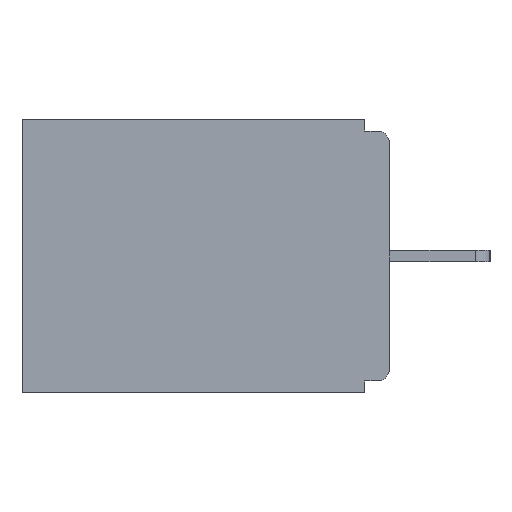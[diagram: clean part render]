
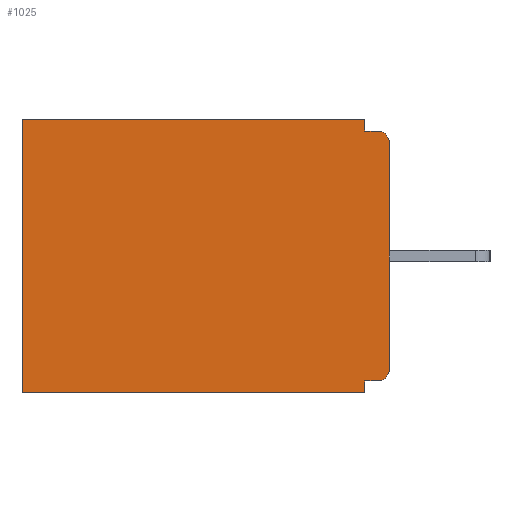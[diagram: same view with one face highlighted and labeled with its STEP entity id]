
A CAD part, left-side view. The second image highlights one B-rep face of the part: STEP entity #1025.
In plain terms, the highlighted planar face has unit normal (-1, 0, 0).
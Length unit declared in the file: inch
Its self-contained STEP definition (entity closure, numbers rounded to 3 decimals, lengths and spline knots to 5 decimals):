
#90 = DIRECTION ( 'NONE',  ( -1., 0., 0. ) ) ;
#140 = VERTEX_POINT ( 'NONE', #8402 ) ;
#780 = PLANE ( 'NONE',  #2413 ) ;
#1025 = ADVANCED_FACE ( 'NONE', ( #2473 ), #780, .F. ) ;
#1148 = ORIENTED_EDGE ( 'NONE', *, *, #9684, .F. ) ;
#1150 = CIRCLE ( 'NONE', #8399, 0.015 ) ;
#1381 = ORIENTED_EDGE ( 'NONE', *, *, #5079, .F. ) ;
#1426 = CARTESIAN_POINT ( 'NONE',  ( 0.298, 0.015, -0.015 ) ) ;
#1466 = CARTESIAN_POINT ( 'NONE',  ( 0.298, 0.46, 0. ) ) ;
#1618 = CARTESIAN_POINT ( 'NONE',  ( 0.298, 0.031, 0. ) ) ;
#1628 = LINE ( 'NONE', #2643, #5589 ) ;
#1726 = DIRECTION ( 'NONE',  ( 0., 0., -1. ) ) ;
#1770 = CARTESIAN_POINT ( 'NONE',  ( 0.298, 0., 0. ) ) ;
#1926 = DIRECTION ( 'NONE',  ( 0., 0., -1. ) ) ;
#1982 = DIRECTION ( 'NONE',  ( 0., 0., -1. ) ) ;
#2405 = EDGE_CURVE ( 'NONE', #10383, #9832, #1628, .T. ) ;
#2413 = AXIS2_PLACEMENT_3D ( 'NONE', #1770, #3349, #8975 ) ;
#2473 = FACE_OUTER_BOUND ( 'NONE', #10370, .T. ) ;
#2510 = VECTOR ( 'NONE', #2753, 39.37008 ) ;
#2528 = LINE ( 'NONE', #3517, #10357 ) ;
#2636 = DIRECTION ( 'NONE',  ( -1., 0., 0. ) ) ;
#2643 = CARTESIAN_POINT ( 'NONE',  ( 0.298, 0., 0. ) ) ;
#2753 = DIRECTION ( 'NONE',  ( 0., 1., 0. ) ) ;
#2997 = VERTEX_POINT ( 'NONE', #1426 ) ;
#3053 = VECTOR ( 'NONE', #3147, 39.37008 ) ;
#3096 = CARTESIAN_POINT ( 'NONE',  ( 0.298, 0.031, -0.343 ) ) ;
#3147 = DIRECTION ( 'NONE',  ( 0., 0., -1. ) ) ;
#3223 = CIRCLE ( 'NONE', #4606, 0.015 ) ;
#3302 = CARTESIAN_POINT ( 'NONE',  ( 0.298, 0.015, -0.313 ) ) ;
#3349 = DIRECTION ( 'NONE',  ( 1., 0., 0. ) ) ;
#3392 = VECTOR ( 'NONE', #7634, 39.37008 ) ;
#3405 = DIRECTION ( 'NONE',  ( 0., 1., 0. ) ) ;
#3458 = DIRECTION ( 'NONE',  ( 0., 0., -1. ) ) ;
#3517 = CARTESIAN_POINT ( 'NONE',  ( 0.298, 0., -0.328 ) ) ;
#3888 = ORIENTED_EDGE ( 'NONE', *, *, #7380, .F. ) ;
#3899 = CARTESIAN_POINT ( 'NONE',  ( 0.298, 0., -0.015 ) ) ;
#3976 = EDGE_CURVE ( 'NONE', #4543, #2997, #9783, .T. ) ;
#4035 = EDGE_CURVE ( 'NONE', #5970, #140, #3223, .T. ) ;
#4049 = CARTESIAN_POINT ( 'NONE',  ( 0.298, 0.015, -0.03 ) ) ;
#4076 = VECTOR ( 'NONE', #8868, 39.37008 ) ;
#4292 = VECTOR ( 'NONE', #1982, 39.37008 ) ;
#4335 = CARTESIAN_POINT ( 'NONE',  ( 0.298, 0.46, 0. ) ) ;
#4396 = EDGE_CURVE ( 'NONE', #5970, #9543, #2528, .T. ) ;
#4543 = VERTEX_POINT ( 'NONE', #5547 ) ;
#4606 = AXIS2_PLACEMENT_3D ( 'NONE', #3302, #2636, #1726 ) ;
#4848 = ORIENTED_EDGE ( 'NONE', *, *, #4035, .T. ) ;
#4960 = VERTEX_POINT ( 'NONE', #5219 ) ;
#5079 = EDGE_CURVE ( 'NONE', #5757, #140, #9377, .T. ) ;
#5086 = DIRECTION ( 'NONE',  ( 0., 1., 0. ) ) ;
#5155 = VECTOR ( 'NONE', #1926, 39.37008 ) ;
#5175 = CARTESIAN_POINT ( 'NONE',  ( 0.298, 0.015, -0.328 ) ) ;
#5198 = ORIENTED_EDGE ( 'NONE', *, *, #9159, .T. ) ;
#5219 = CARTESIAN_POINT ( 'NONE',  ( 0.298, 0.46, -0.343 ) ) ;
#5221 = LINE ( 'NONE', #5334, #5155 ) ;
#5334 = CARTESIAN_POINT ( 'NONE',  ( 0.298, 0.031, -0.343 ) ) ;
#5380 = CARTESIAN_POINT ( 'NONE',  ( 0.298, 0., 0. ) ) ;
#5547 = CARTESIAN_POINT ( 'NONE',  ( 0.298, 0.031, -0.015 ) ) ;
#5589 = VECTOR ( 'NONE', #5086, 39.37008 ) ;
#5757 = VERTEX_POINT ( 'NONE', #6188 ) ;
#5771 = EDGE_CURVE ( 'NONE', #9832, #4960, #7889, .T. ) ;
#5918 = ORIENTED_EDGE ( 'NONE', *, *, #2405, .T. ) ;
#5970 = VERTEX_POINT ( 'NONE', #5175 ) ;
#6044 = CARTESIAN_POINT ( 'NONE',  ( 0.298, 0.031, -0.343 ) ) ;
#6188 = CARTESIAN_POINT ( 'NONE',  ( 0.298, 0., -0.03 ) ) ;
#6507 = CARTESIAN_POINT ( 'NONE',  ( 0.298, 0.031, -0.328 ) ) ;
#6909 = VERTEX_POINT ( 'NONE', #6044 ) ;
#7308 = LINE ( 'NONE', #3096, #3053 ) ;
#7380 = EDGE_CURVE ( 'NONE', #6909, #4960, #7675, .T. ) ;
#7469 = ORIENTED_EDGE ( 'NONE', *, *, #4396, .F. ) ;
#7634 = DIRECTION ( 'NONE',  ( 0., 0., -1. ) ) ;
#7675 = LINE ( 'NONE', #10209, #2510 ) ;
#7889 = LINE ( 'NONE', #4335, #3392 ) ;
#8282 = EDGE_CURVE ( 'NONE', #9543, #6909, #7308, .T. ) ;
#8399 = AXIS2_PLACEMENT_3D ( 'NONE', #4049, #90, #3458 ) ;
#8402 = CARTESIAN_POINT ( 'NONE',  ( 0.298, 0., -0.313 ) ) ;
#8627 = ORIENTED_EDGE ( 'NONE', *, *, #8282, .F. ) ;
#8868 = DIRECTION ( 'NONE',  ( 0., -1., 0. ) ) ;
#8975 = DIRECTION ( 'NONE',  ( 0., 0., -1. ) ) ;
#9159 = EDGE_CURVE ( 'NONE', #5757, #2997, #1150, .T. ) ;
#9377 = LINE ( 'NONE', #5380, #4292 ) ;
#9543 = VERTEX_POINT ( 'NONE', #6507 ) ;
#9587 = ORIENTED_EDGE ( 'NONE', *, *, #5771, .T. ) ;
#9684 = EDGE_CURVE ( 'NONE', #10383, #4543, #5221, .T. ) ;
#9783 = LINE ( 'NONE', #3899, #4076 ) ;
#9832 = VERTEX_POINT ( 'NONE', #1466 ) ;
#9962 = ORIENTED_EDGE ( 'NONE', *, *, #3976, .F. ) ;
#10209 = CARTESIAN_POINT ( 'NONE',  ( 0.298, 0., -0.343 ) ) ;
#10357 = VECTOR ( 'NONE', #3405, 39.37008 ) ;
#10370 = EDGE_LOOP ( 'NONE', ( #5198, #9962, #1148, #5918, #9587, #3888, #8627, #7469, #4848, #1381 ) ) ;
#10383 = VERTEX_POINT ( 'NONE', #1618 ) ;
